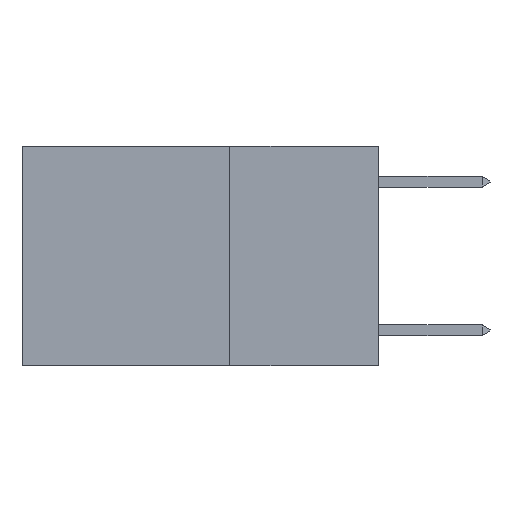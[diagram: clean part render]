
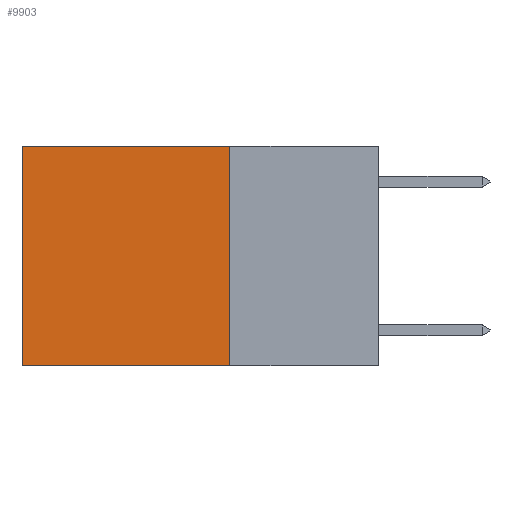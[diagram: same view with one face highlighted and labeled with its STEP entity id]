
A CAD part, left-side view. The second image highlights one B-rep face of the part: STEP entity #9903.
In plain terms, the highlighted planar face has unit normal (-1, 0, 0).
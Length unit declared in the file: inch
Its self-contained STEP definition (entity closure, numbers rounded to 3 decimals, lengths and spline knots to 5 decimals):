
#1861 = VECTOR ( 'NONE', #2133, 39.37008 ) ;
#2131 = DIRECTION ( 'NONE',  ( 0., 0., -1. ) ) ;
#2133 = DIRECTION ( 'NONE',  ( 0., 0., -1. ) ) ;
#2504 = EDGE_CURVE ( 'NONE', #2753, #3277, #4118, .T. ) ;
#2753 = VERTEX_POINT ( 'NONE', #7435 ) ;
#3051 = EDGE_CURVE ( 'NONE', #17791, #8039, #20852, .T. ) ;
#3277 = VERTEX_POINT ( 'NONE', #9833 ) ;
#3308 = FACE_OUTER_BOUND ( 'NONE', #13883, .T. ) ;
#3385 = CARTESIAN_POINT ( 'NONE',  ( 0.2625, 0.6, -0.37 ) ) ;
#3439 = ORIENTED_EDGE ( 'NONE', *, *, #2504, .T. ) ;
#3530 = DIRECTION ( 'NONE',  ( 1., 0., 0. ) ) ;
#4118 = LINE ( 'NONE', #8152, #15976 ) ;
#5322 = VECTOR ( 'NONE', #19103, 39.37008 ) ;
#5802 = LINE ( 'NONE', #5929, #1861 ) ;
#5929 = CARTESIAN_POINT ( 'NONE',  ( 0.2625, 0.25, 0. ) ) ;
#7435 = CARTESIAN_POINT ( 'NONE',  ( 0.2625, 0.25, 0. ) ) ;
#8039 = VERTEX_POINT ( 'NONE', #3385 ) ;
#8152 = CARTESIAN_POINT ( 'NONE',  ( 0.2625, 0.25, 0. ) ) ;
#9833 = CARTESIAN_POINT ( 'NONE',  ( 0.2625, 0.6, 0. ) ) ;
#9903 = ADVANCED_FACE ( 'NONE', ( #3308 ), #19266, .F. ) ;
#10139 = EDGE_CURVE ( 'NONE', #3277, #8039, #11075, .T. ) ;
#11075 = LINE ( 'NONE', #18312, #23123 ) ;
#13484 = ORIENTED_EDGE ( 'NONE', *, *, #10139, .T. ) ;
#13715 = CARTESIAN_POINT ( 'NONE',  ( 0.2625, 0.25, -0.37 ) ) ;
#13878 = CARTESIAN_POINT ( 'NONE',  ( 0.2625, 0.25, -0.37 ) ) ;
#13883 = EDGE_LOOP ( 'NONE', ( #13484, #21110, #14417, #3439 ) ) ;
#14417 = ORIENTED_EDGE ( 'NONE', *, *, #17988, .F. ) ;
#15347 = DIRECTION ( 'NONE',  ( 0., 1., 0. ) ) ;
#15976 = VECTOR ( 'NONE', #15347, 39.37008 ) ;
#17719 = DIRECTION ( 'NONE',  ( 0., 0., -1. ) ) ;
#17791 = VERTEX_POINT ( 'NONE', #13715 ) ;
#17988 = EDGE_CURVE ( 'NONE', #2753, #17791, #5802, .T. ) ;
#18312 = CARTESIAN_POINT ( 'NONE',  ( 0.2625, 0.6, 0. ) ) ;
#18619 = AXIS2_PLACEMENT_3D ( 'NONE', #19386, #3530, #17719 ) ;
#19103 = DIRECTION ( 'NONE',  ( 0., 1., 0. ) ) ;
#19266 = PLANE ( 'NONE',  #18619 ) ;
#19386 = CARTESIAN_POINT ( 'NONE',  ( 0.2625, 0.25, 0. ) ) ;
#20852 = LINE ( 'NONE', #13878, #5322 ) ;
#21110 = ORIENTED_EDGE ( 'NONE', *, *, #3051, .F. ) ;
#23123 = VECTOR ( 'NONE', #2131, 39.37008 ) ;
